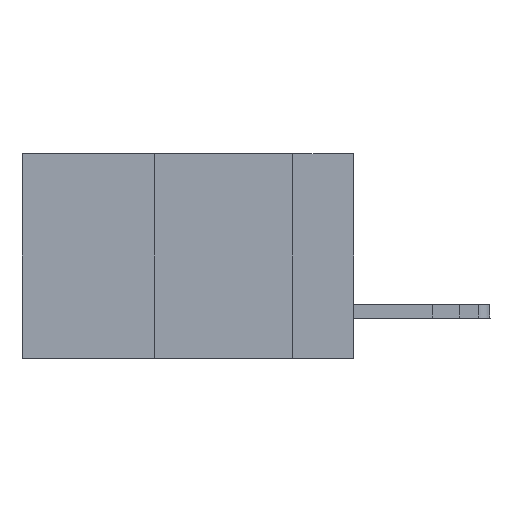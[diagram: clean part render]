
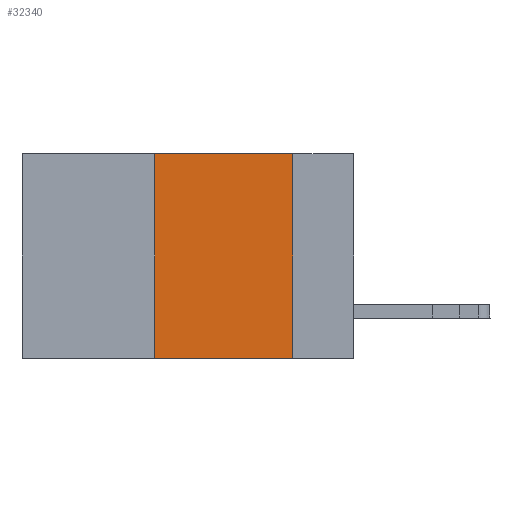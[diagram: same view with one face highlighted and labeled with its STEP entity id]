
A CAD part, left-side view. The second image highlights one B-rep face of the part: STEP entity #32340.
In plain terms, the highlighted planar face has unit normal (-1, 0, 0).
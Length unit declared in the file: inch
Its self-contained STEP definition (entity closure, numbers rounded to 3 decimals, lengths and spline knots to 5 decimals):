
#884 = VECTOR ( 'NONE', #25347, 39.37008 ) ;
#3169 = CARTESIAN_POINT ( 'NONE',  ( 0., 0.36, 0. ) ) ;
#3652 = EDGE_LOOP ( 'NONE', ( #15794, #7997, #5521, #32368 ) ) ;
#4772 = CARTESIAN_POINT ( 'NONE',  ( 0., 0.36, 0. ) ) ;
#5347 = LINE ( 'NONE', #3169, #25417 ) ;
#5429 = VERTEX_POINT ( 'NONE', #22196 ) ;
#5521 = ORIENTED_EDGE ( 'NONE', *, *, #27162, .F. ) ;
#5742 = DIRECTION ( 'NONE',  ( 0., -1., 0. ) ) ;
#7116 = DIRECTION ( 'NONE',  ( 0., 0., -1. ) ) ;
#7801 = VERTEX_POINT ( 'NONE', #11039 ) ;
#7997 = ORIENTED_EDGE ( 'NONE', *, *, #18849, .F. ) ;
#9101 = VECTOR ( 'NONE', #7116, 39.37008 ) ;
#9336 = EDGE_CURVE ( 'NONE', #5429, #22132, #28140, .T. ) ;
#9792 = CARTESIAN_POINT ( 'NONE',  ( 0., 0.11, 0. ) ) ;
#11039 = CARTESIAN_POINT ( 'NONE',  ( 0., 0.11, 0. ) ) ;
#12526 = CARTESIAN_POINT ( 'NONE',  ( 0., 0.6, 0. ) ) ;
#12655 = CARTESIAN_POINT ( 'NONE',  ( 0., 0.11, -0.37 ) ) ;
#12702 = FACE_OUTER_BOUND ( 'NONE', #3652, .T. ) ;
#12866 = VECTOR ( 'NONE', #5742, 39.37008 ) ;
#15337 = DIRECTION ( 'NONE',  ( 0., 0., -1. ) ) ;
#15794 = ORIENTED_EDGE ( 'NONE', *, *, #16022, .F. ) ;
#15929 = AXIS2_PLACEMENT_3D ( 'NONE', #12526, #31539, #15337 ) ;
#16022 = EDGE_CURVE ( 'NONE', #7801, #22132, #16473, .T. ) ;
#16473 = LINE ( 'NONE', #9792, #9101 ) ;
#17080 = CARTESIAN_POINT ( 'NONE',  ( 0., 0.6, -0.37 ) ) ;
#18849 = EDGE_CURVE ( 'NONE', #32966, #7801, #23686, .T. ) ;
#19826 = CARTESIAN_POINT ( 'NONE',  ( 0., 0.6, 0. ) ) ;
#22132 = VERTEX_POINT ( 'NONE', #12655 ) ;
#22196 = CARTESIAN_POINT ( 'NONE',  ( 0., 0.36, -0.37 ) ) ;
#23686 = LINE ( 'NONE', #19826, #884 ) ;
#25347 = DIRECTION ( 'NONE',  ( 0., -1., 0. ) ) ;
#25417 = VECTOR ( 'NONE', #33223, 39.37008 ) ;
#27162 = EDGE_CURVE ( 'NONE', #5429, #32966, #5347, .T. ) ;
#28140 = LINE ( 'NONE', #17080, #12866 ) ;
#31539 = DIRECTION ( 'NONE',  ( 1., 0., 0. ) ) ;
#32340 = ADVANCED_FACE ( 'NONE', ( #12702 ), #34809, .F. ) ;
#32368 = ORIENTED_EDGE ( 'NONE', *, *, #9336, .T. ) ;
#32966 = VERTEX_POINT ( 'NONE', #4772 ) ;
#33223 = DIRECTION ( 'NONE',  ( 0., 0., 1. ) ) ;
#34809 = PLANE ( 'NONE',  #15929 ) ;
